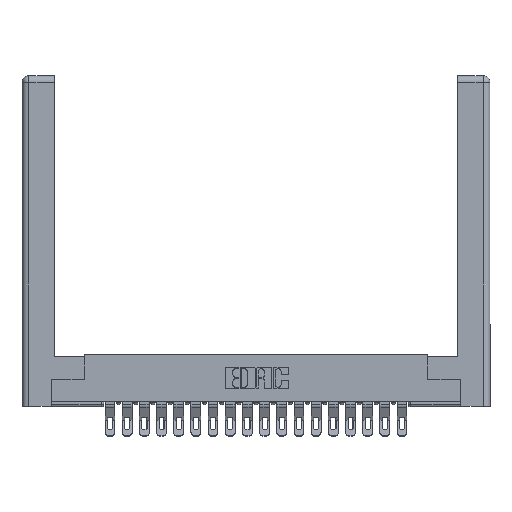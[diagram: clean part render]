
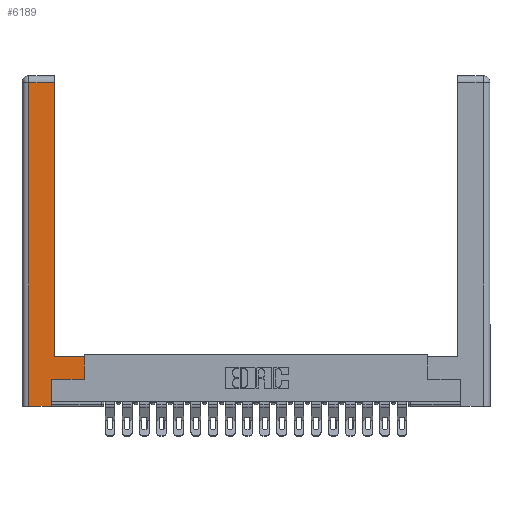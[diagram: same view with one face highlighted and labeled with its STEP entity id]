
A CAD part, top view. The second image highlights one B-rep face of the part: STEP entity #6189.
In plain terms, the highlighted planar face has unit normal (0, 0, 1).
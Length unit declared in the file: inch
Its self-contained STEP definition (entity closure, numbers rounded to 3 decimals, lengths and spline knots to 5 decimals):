
#274 = CARTESIAN_POINT ( 'NONE',  ( 0.565, 0.45, 0. ) ) ;
#605 = ORIENTED_EDGE ( 'NONE', *, *, #18786, .T. ) ;
#826 = CARTESIAN_POINT ( 'NONE',  ( 0.0615, 0., 0. ) ) ;
#1029 = CARTESIAN_POINT ( 'NONE',  ( 0.295, 2.94, 0. ) ) ;
#1084 = DIRECTION ( 'NONE',  ( 0., 1., 0. ) ) ;
#1154 = CARTESIAN_POINT ( 'NONE',  ( 0.295, 3., 0. ) ) ;
#4218 = VERTEX_POINT ( 'NONE', #1029 ) ;
#4630 = EDGE_LOOP ( 'NONE', ( #605, #11620, #6800, #17152, #7052, #18520, #4781, #8968 ) ) ;
#4781 = ORIENTED_EDGE ( 'NONE', *, *, #10713, .T. ) ;
#5132 = CARTESIAN_POINT ( 'NONE',  ( 0., 0., 0. ) ) ;
#5807 = CARTESIAN_POINT ( 'NONE',  ( 0.0615, 2.94, 0. ) ) ;
#5810 = VERTEX_POINT ( 'NONE', #5946 ) ;
#5946 = CARTESIAN_POINT ( 'NONE',  ( 0.565, 0.45, 0. ) ) ;
#6189 = ADVANCED_FACE ( 'NONE', ( #15337 ), #18913, .F. ) ;
#6262 = EDGE_CURVE ( 'NONE', #16283, #17936, #21935, .T. ) ;
#6271 = VECTOR ( 'NONE', #1084, 39.37008 ) ;
#6800 = ORIENTED_EDGE ( 'NONE', *, *, #13111, .T. ) ;
#7040 = DIRECTION ( 'NONE',  ( -1., 0., 0. ) ) ;
#7052 = ORIENTED_EDGE ( 'NONE', *, *, #6262, .T. ) ;
#7644 = LINE ( 'NONE', #21393, #13942 ) ;
#8837 = EDGE_CURVE ( 'NONE', #10388, #16283, #9384, .T. ) ;
#8968 = ORIENTED_EDGE ( 'NONE', *, *, #19602, .T. ) ;
#9261 = CARTESIAN_POINT ( 'NONE',  ( 0.565, 0.245, 0. ) ) ;
#9350 = DIRECTION ( 'NONE',  ( 0., 1., 0. ) ) ;
#9384 = LINE ( 'NONE', #11613, #18799 ) ;
#9513 = LINE ( 'NONE', #11192, #10590 ) ;
#10388 = VERTEX_POINT ( 'NONE', #826 ) ;
#10590 = VECTOR ( 'NONE', #16014, 39.37008 ) ;
#10688 = CARTESIAN_POINT ( 'NONE',  ( 0.565, 0.245, 0. ) ) ;
#10713 = EDGE_CURVE ( 'NONE', #14058, #5810, #20887, .T. ) ;
#11192 = CARTESIAN_POINT ( 'NONE',  ( 0.295, 0.45, 0. ) ) ;
#11279 = DIRECTION ( 'NONE',  ( 1., 0., 0. ) ) ;
#11386 = VECTOR ( 'NONE', #19093, 39.37008 ) ;
#11613 = CARTESIAN_POINT ( 'NONE',  ( 0.265, 0., 0. ) ) ;
#11620 = ORIENTED_EDGE ( 'NONE', *, *, #14635, .T. ) ;
#11709 = VECTOR ( 'NONE', #15405, 39.37008 ) ;
#11966 = DIRECTION ( 'NONE',  ( -1., 0., 0. ) ) ;
#12446 = CARTESIAN_POINT ( 'NONE',  ( 0.0615, 2.94, 0. ) ) ;
#12562 = CARTESIAN_POINT ( 'NONE',  ( 0.295, 0.45, 0. ) ) ;
#13057 = CARTESIAN_POINT ( 'NONE',  ( 0.265, 0.245, 0. ) ) ;
#13111 = EDGE_CURVE ( 'NONE', #17164, #10388, #7644, .T. ) ;
#13942 = VECTOR ( 'NONE', #14447, 39.37008 ) ;
#14058 = VERTEX_POINT ( 'NONE', #9261 ) ;
#14084 = LINE ( 'NONE', #5807, #20744 ) ;
#14447 = DIRECTION ( 'NONE',  ( 0., -1., 0. ) ) ;
#14507 = CARTESIAN_POINT ( 'NONE',  ( 0.265, 0., 0. ) ) ;
#14635 = EDGE_CURVE ( 'NONE', #4218, #17164, #14084, .T. ) ;
#15278 = AXIS2_PLACEMENT_3D ( 'NONE', #5132, #18487, #11966 ) ;
#15337 = FACE_OUTER_BOUND ( 'NONE', #4630, .T. ) ;
#15405 = DIRECTION ( 'NONE',  ( 1., 0., 0. ) ) ;
#15573 = VECTOR ( 'NONE', #9350, 39.37008 ) ;
#15618 = LINE ( 'NONE', #10688, #11709 ) ;
#16014 = DIRECTION ( 'NONE',  ( -1., 0., 0. ) ) ;
#16283 = VERTEX_POINT ( 'NONE', #14507 ) ;
#17152 = ORIENTED_EDGE ( 'NONE', *, *, #8837, .T. ) ;
#17164 = VERTEX_POINT ( 'NONE', #12446 ) ;
#17936 = VERTEX_POINT ( 'NONE', #19426 ) ;
#18297 = VERTEX_POINT ( 'NONE', #12562 ) ;
#18487 = DIRECTION ( 'NONE',  ( 0., 0., -1. ) ) ;
#18520 = ORIENTED_EDGE ( 'NONE', *, *, #20363, .T. ) ;
#18786 = EDGE_CURVE ( 'NONE', #18297, #4218, #19643, .T. ) ;
#18799 = VECTOR ( 'NONE', #11279, 39.37008 ) ;
#18913 = PLANE ( 'NONE',  #15278 ) ;
#19093 = DIRECTION ( 'NONE',  ( 0., 1., 0. ) ) ;
#19426 = CARTESIAN_POINT ( 'NONE',  ( 0.265, 0.245, 0. ) ) ;
#19602 = EDGE_CURVE ( 'NONE', #5810, #18297, #9513, .T. ) ;
#19643 = LINE ( 'NONE', #1154, #15573 ) ;
#20363 = EDGE_CURVE ( 'NONE', #17936, #14058, #15618, .T. ) ;
#20744 = VECTOR ( 'NONE', #7040, 39.37008 ) ;
#20887 = LINE ( 'NONE', #274, #11386 ) ;
#21393 = CARTESIAN_POINT ( 'NONE',  ( 0.0615, 0., 0. ) ) ;
#21935 = LINE ( 'NONE', #13057, #6271 ) ;
